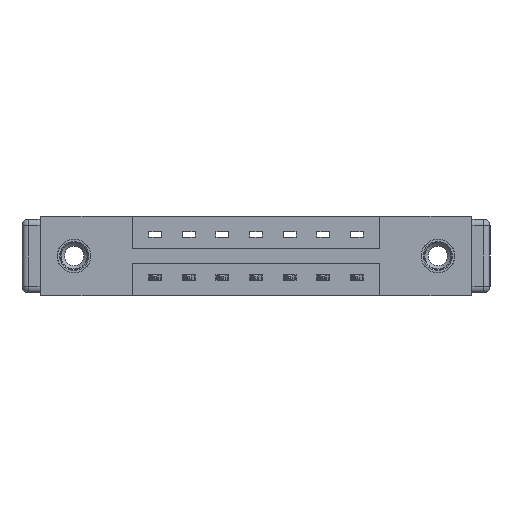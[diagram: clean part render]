
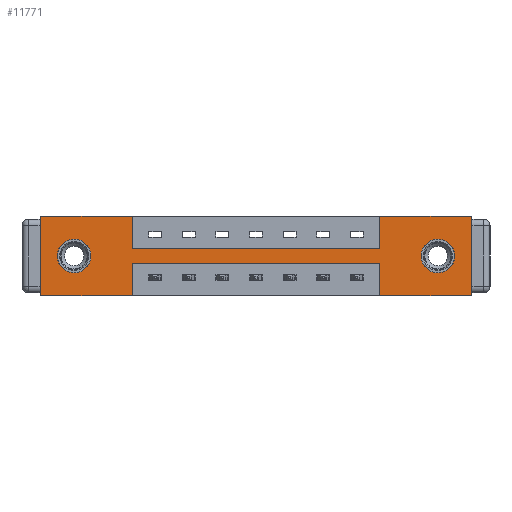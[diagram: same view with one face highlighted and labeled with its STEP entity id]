
A CAD part, front view. The second image highlights one B-rep face of the part: STEP entity #11771.
In plain terms, the highlighted planar face has unit normal (0, -1, 0).
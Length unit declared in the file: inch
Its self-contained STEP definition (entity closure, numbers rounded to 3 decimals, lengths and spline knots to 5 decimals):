
#99 = VERTEX_POINT ( 'NONE', #3029 ) ;
#173 = VERTEX_POINT ( 'NONE', #7573 ) ;
#244 = LINE ( 'NONE', #8267, #8225 ) ;
#287 = DIRECTION ( 'NONE',  ( 0., 0., -1. ) ) ;
#511 = CARTESIAN_POINT ( 'NONE',  ( 0., 0., -0.37 ) ) ;
#658 = CARTESIAN_POINT ( 'NONE',  ( 0.155, 0., -0.263 ) ) ;
#690 = DIRECTION ( 'NONE',  ( 0., 0., 1. ) ) ;
#728 = DIRECTION ( 'NONE',  ( 1., 0., 0. ) ) ;
#801 = VERTEX_POINT ( 'NONE', #9347 ) ;
#861 = AXIS2_PLACEMENT_3D ( 'NONE', #7126, #8979, #10080 ) ;
#948 = VERTEX_POINT ( 'NONE', #11843 ) ;
#994 = VERTEX_POINT ( 'NONE', #9883 ) ;
#1014 = EDGE_CURVE ( 'NONE', #99, #10993, #4403, .T. ) ;
#1167 = VECTOR ( 'NONE', #6454, 39.37008 ) ;
#1248 = EDGE_CURVE ( 'NONE', #6469, #8367, #6951, .T. ) ;
#1317 = VERTEX_POINT ( 'NONE', #4395 ) ;
#1320 = ORIENTED_EDGE ( 'NONE', *, *, #7617, .T. ) ;
#1425 = LINE ( 'NONE', #1636, #9119 ) ;
#1636 = CARTESIAN_POINT ( 'NONE',  ( 0., 0., -0.37 ) ) ;
#1906 = VECTOR ( 'NONE', #690, 39.37008 ) ;
#2246 = LINE ( 'NONE', #12176, #8276 ) ;
#2371 = FACE_OUTER_BOUND ( 'NONE', #8271, .T. ) ;
#2419 = EDGE_CURVE ( 'NONE', #948, #99, #6458, .T. ) ;
#2526 = FACE_BOUND ( 'NONE', #7026, .T. ) ;
#2529 = CARTESIAN_POINT ( 'NONE',  ( 0., 0., -0.37 ) ) ;
#2538 = DIRECTION ( 'NONE',  ( 1., 0., 0. ) ) ;
#2922 = EDGE_CURVE ( 'NONE', #10993, #3634, #7024, .T. ) ;
#3024 = EDGE_CURVE ( 'NONE', #994, #7251, #244, .T. ) ;
#3029 = CARTESIAN_POINT ( 'NONE',  ( 0.425, 0., 0. ) ) ;
#3383 = VERTEX_POINT ( 'NONE', #511 ) ;
#3432 = LINE ( 'NONE', #12317, #1906 ) ;
#3508 = ORIENTED_EDGE ( 'NONE', *, *, #8988, .T. ) ;
#3524 = DIRECTION ( 'NONE',  ( 0., -1., 0. ) ) ;
#3587 = LINE ( 'NONE', #8329, #1167 ) ;
#3591 = EDGE_CURVE ( 'NONE', #801, #3383, #1425, .T. ) ;
#3634 = VERTEX_POINT ( 'NONE', #10462 ) ;
#3635 = VERTEX_POINT ( 'NONE', #10584 ) ;
#3824 = CARTESIAN_POINT ( 'NONE',  ( 1.843, 0., -0.185 ) ) ;
#3852 = ORIENTED_EDGE ( 'NONE', *, *, #2922, .F. ) ;
#3935 = EDGE_CURVE ( 'NONE', #7251, #801, #5346, .T. ) ;
#4021 = VERTEX_POINT ( 'NONE', #8111 ) ;
#4102 = VECTOR ( 'NONE', #6421, 39.37008 ) ;
#4329 = FACE_BOUND ( 'NONE', #5103, .T. ) ;
#4335 = ORIENTED_EDGE ( 'NONE', *, *, #1014, .F. ) ;
#4373 = ORIENTED_EDGE ( 'NONE', *, *, #9009, .F. ) ;
#4395 = CARTESIAN_POINT ( 'NONE',  ( 1.998, 0., 0. ) ) ;
#4403 = LINE ( 'NONE', #5076, #11499 ) ;
#4543 = LINE ( 'NONE', #8297, #4102 ) ;
#4614 = ORIENTED_EDGE ( 'NONE', *, *, #9838, .T. ) ;
#5076 = CARTESIAN_POINT ( 'NONE',  ( 0.425, 0., 0. ) ) ;
#5103 = EDGE_LOOP ( 'NONE', ( #9281, #3508 ) ) ;
#5346 = LINE ( 'NONE', #11941, #8649 ) ;
#5394 = CARTESIAN_POINT ( 'NONE',  ( 0.425, 0., -0.15 ) ) ;
#5409 = CIRCLE ( 'NONE', #861, 0.078 ) ;
#5463 = LINE ( 'NONE', #8965, #10758 ) ;
#5534 = CARTESIAN_POINT ( 'NONE',  ( 0., 0., 0. ) ) ;
#5536 = EDGE_CURVE ( 'NONE', #4021, #994, #4543, .T. ) ;
#5572 = CARTESIAN_POINT ( 'NONE',  ( 0.425, 0., -0.22 ) ) ;
#5601 = VERTEX_POINT ( 'NONE', #9447 ) ;
#5753 = DIRECTION ( 'NONE',  ( 0., 1., 0. ) ) ;
#5996 = ORIENTED_EDGE ( 'NONE', *, *, #2419, .F. ) ;
#6012 = DIRECTION ( 'NONE',  ( 0., 0., 1. ) ) ;
#6097 = DIRECTION ( 'NONE',  ( 0., 0., 1. ) ) ;
#6237 = CARTESIAN_POINT ( 'NONE',  ( 1.843, 0., -0.107 ) ) ;
#6263 = ORIENTED_EDGE ( 'NONE', *, *, #3591, .F. ) ;
#6360 = PLANE ( 'NONE',  #10320 ) ;
#6421 = DIRECTION ( 'NONE',  ( 0., 0., 1. ) ) ;
#6454 = DIRECTION ( 'NONE',  ( 0., 0., -1. ) ) ;
#6458 = LINE ( 'NONE', #5534, #9760 ) ;
#6469 = VERTEX_POINT ( 'NONE', #8499 ) ;
#6515 = DIRECTION ( 'NONE',  ( 1., 0., 0. ) ) ;
#6795 = VECTOR ( 'NONE', #10695, 39.37008 ) ;
#6810 = ORIENTED_EDGE ( 'NONE', *, *, #7240, .F. ) ;
#6951 = CIRCLE ( 'NONE', #9609, 0.078 ) ;
#7023 = DIRECTION ( 'NONE',  ( 0., 1., 0. ) ) ;
#7024 = LINE ( 'NONE', #8293, #7331 ) ;
#7026 = EDGE_LOOP ( 'NONE', ( #1320, #4614 ) ) ;
#7126 = CARTESIAN_POINT ( 'NONE',  ( 1.843, 0., -0.185 ) ) ;
#7225 = CARTESIAN_POINT ( 'NONE',  ( 0.155, 0., -0.185 ) ) ;
#7240 = EDGE_CURVE ( 'NONE', #5601, #1317, #2246, .T. ) ;
#7251 = VERTEX_POINT ( 'NONE', #5572 ) ;
#7331 = VECTOR ( 'NONE', #2538, 39.37008 ) ;
#7345 = ORIENTED_EDGE ( 'NONE', *, *, #3024, .F. ) ;
#7573 = CARTESIAN_POINT ( 'NONE',  ( 1.998, 0., -0.37 ) ) ;
#7617 = EDGE_CURVE ( 'NONE', #10418, #3635, #5409, .T. ) ;
#7663 = ORIENTED_EDGE ( 'NONE', *, *, #10997, .F. ) ;
#7680 = CARTESIAN_POINT ( 'NONE',  ( 0., 0., -0.37 ) ) ;
#7687 = LINE ( 'NONE', #7680, #6795 ) ;
#8010 = CIRCLE ( 'NONE', #10195, 0.078 ) ;
#8111 = CARTESIAN_POINT ( 'NONE',  ( 1.573, 0., -0.37 ) ) ;
#8225 = VECTOR ( 'NONE', #12224, 39.37008 ) ;
#8267 = CARTESIAN_POINT ( 'NONE',  ( 0.425, 0., -0.22 ) ) ;
#8271 = EDGE_LOOP ( 'NONE', ( #10954, #7345, #10579, #8442, #7663, #6810, #11331, #3852, #4335, #5996, #4373, #6263 ) ) ;
#8276 = VECTOR ( 'NONE', #6515, 39.37008 ) ;
#8293 = CARTESIAN_POINT ( 'NONE',  ( 0.425, 0., -0.15 ) ) ;
#8297 = CARTESIAN_POINT ( 'NONE',  ( 1.573, 0., -0.37 ) ) ;
#8329 = CARTESIAN_POINT ( 'NONE',  ( 1.998, 0., 0. ) ) ;
#8346 = DIRECTION ( 'NONE',  ( 0., 1., 0. ) ) ;
#8367 = VERTEX_POINT ( 'NONE', #658 ) ;
#8442 = ORIENTED_EDGE ( 'NONE', *, *, #9803, .F. ) ;
#8499 = CARTESIAN_POINT ( 'NONE',  ( 0.155, 0., -0.107 ) ) ;
#8649 = VECTOR ( 'NONE', #287, 39.37008 ) ;
#8965 = CARTESIAN_POINT ( 'NONE',  ( 0., 0., 0. ) ) ;
#8979 = DIRECTION ( 'NONE',  ( 0., 1., 0. ) ) ;
#8988 = EDGE_CURVE ( 'NONE', #8367, #6469, #8010, .T. ) ;
#9009 = EDGE_CURVE ( 'NONE', #3383, #948, #5463, .T. ) ;
#9119 = VECTOR ( 'NONE', #12254, 39.37008 ) ;
#9248 = DIRECTION ( 'NONE',  ( 0., 0., 1. ) ) ;
#9281 = ORIENTED_EDGE ( 'NONE', *, *, #1248, .T. ) ;
#9347 = CARTESIAN_POINT ( 'NONE',  ( 0.425, 0., -0.37 ) ) ;
#9447 = CARTESIAN_POINT ( 'NONE',  ( 1.573, 0., 0. ) ) ;
#9460 = AXIS2_PLACEMENT_3D ( 'NONE', #3824, #5753, #10654 ) ;
#9609 = AXIS2_PLACEMENT_3D ( 'NONE', #7225, #8346, #9248 ) ;
#9760 = VECTOR ( 'NONE', #728, 39.37008 ) ;
#9803 = EDGE_CURVE ( 'NONE', #173, #4021, #7687, .T. ) ;
#9838 = EDGE_CURVE ( 'NONE', #3635, #10418, #11327, .T. ) ;
#9883 = CARTESIAN_POINT ( 'NONE',  ( 1.573, 0., -0.22 ) ) ;
#10080 = DIRECTION ( 'NONE',  ( 0., 0., -1. ) ) ;
#10195 = AXIS2_PLACEMENT_3D ( 'NONE', #10869, #7023, #6097 ) ;
#10320 = AXIS2_PLACEMENT_3D ( 'NONE', #2529, #3524, #12284 ) ;
#10418 = VERTEX_POINT ( 'NONE', #6237 ) ;
#10462 = CARTESIAN_POINT ( 'NONE',  ( 1.573, 0., -0.15 ) ) ;
#10579 = ORIENTED_EDGE ( 'NONE', *, *, #5536, .F. ) ;
#10584 = CARTESIAN_POINT ( 'NONE',  ( 1.843, 0., -0.263 ) ) ;
#10654 = DIRECTION ( 'NONE',  ( 0., 0., -1. ) ) ;
#10695 = DIRECTION ( 'NONE',  ( -1., 0., 0. ) ) ;
#10758 = VECTOR ( 'NONE', #6012, 39.37008 ) ;
#10816 = DIRECTION ( 'NONE',  ( 0., 0., -1. ) ) ;
#10869 = CARTESIAN_POINT ( 'NONE',  ( 0.155, 0., -0.185 ) ) ;
#10954 = ORIENTED_EDGE ( 'NONE', *, *, #3935, .F. ) ;
#10993 = VERTEX_POINT ( 'NONE', #5394 ) ;
#10997 = EDGE_CURVE ( 'NONE', #1317, #173, #3587, .T. ) ;
#11327 = CIRCLE ( 'NONE', #9460, 0.078 ) ;
#11331 = ORIENTED_EDGE ( 'NONE', *, *, #11358, .F. ) ;
#11358 = EDGE_CURVE ( 'NONE', #3634, #5601, #3432, .T. ) ;
#11499 = VECTOR ( 'NONE', #10816, 39.37008 ) ;
#11771 = ADVANCED_FACE ( 'NONE', ( #2526, #4329, #2371 ), #6360, .T. ) ;
#11843 = CARTESIAN_POINT ( 'NONE',  ( 0., 0., 0. ) ) ;
#11941 = CARTESIAN_POINT ( 'NONE',  ( 0.425, 0., -0.37 ) ) ;
#12176 = CARTESIAN_POINT ( 'NONE',  ( 0., 0., 0. ) ) ;
#12224 = DIRECTION ( 'NONE',  ( -1., 0., 0. ) ) ;
#12254 = DIRECTION ( 'NONE',  ( -1., 0., 0. ) ) ;
#12284 = DIRECTION ( 'NONE',  ( 0., 0., -1. ) ) ;
#12317 = CARTESIAN_POINT ( 'NONE',  ( 1.573, 0., 0. ) ) ;
